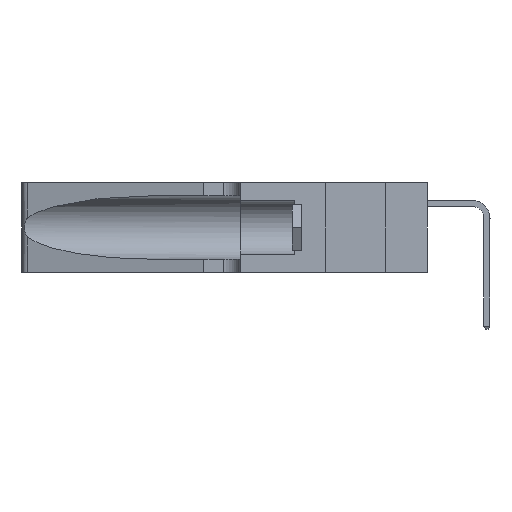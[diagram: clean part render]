
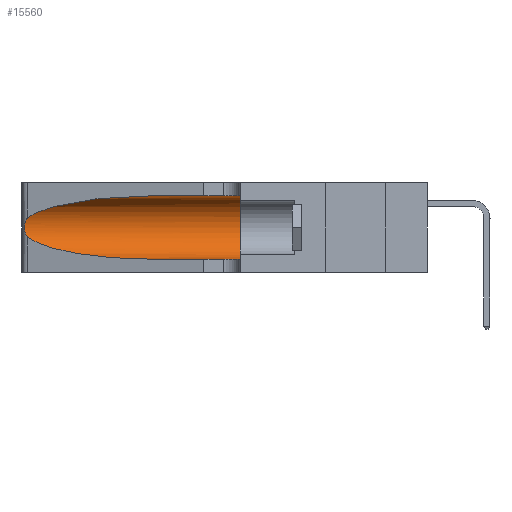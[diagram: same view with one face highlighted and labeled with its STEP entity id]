
A CAD part, left-side view. The second image highlights one B-rep face of the part: STEP entity #15560.
In plain terms, the highlighted cylindrical face has radius 3.308 mm (diameter 6.617 mm), a partial arc.
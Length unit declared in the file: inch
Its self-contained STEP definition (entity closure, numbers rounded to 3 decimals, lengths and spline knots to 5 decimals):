
#307 = CARTESIAN_POINT ( 'NONE',  ( 0.25856, 1.23593, 0.16098 ) ) ;
#1010 = EDGE_CURVE ( 'NONE', #24954, #26851, #30352, .T. ) ;
#1242 = CARTESIAN_POINT ( 'NONE',  ( 0.1305, 0.35, 0.31525 ) ) ;
#2474 = VERTEX_POINT ( 'NONE', #1242 ) ;
#3265 = CARTESIAN_POINT ( 'NONE',  ( 0.25487, 1.22718, 0.22369 ) ) ;
#3398 = CARTESIAN_POINT ( 'NONE',  ( 0.25639, 1.23186, 0.15144 ) ) ;
#3695 = DIRECTION ( 'NONE',  ( 0., 0., -1. ) ) ;
#4111 = VERTEX_POINT ( 'NONE', #16130 ) ;
#4915 = CARTESIAN_POINT ( 'NONE',  ( 0.1305, 0.72297, 0.31525 ) ) ;
#5141 = ORIENTED_EDGE ( 'NONE', *, *, #1010, .T. ) ;
#5657 = CARTESIAN_POINT ( 'NONE',  ( 0.18966, 0.96281, 0.05475 ) ) ;
#6022 = CARTESIAN_POINT ( 'NONE',  ( 0.1305, 0.72297, 0.31525 ) ) ;
#6256 = VECTOR ( 'NONE', #17718, 39.37008 ) ;
#6457 = CARTESIAN_POINT ( 'NONE',  ( 0.25487, 1.22718, 0.14631 ) ) ;
#6634 = CARTESIAN_POINT ( 'NONE',  ( 0.1305, 0.35, 0.05475 ) ) ;
#6890 = AXIS2_PLACEMENT_3D ( 'NONE', #16538, #37881, #19611 ) ;
#8808 = CIRCLE ( 'NONE', #6890, 0.13025 ) ;
#9155 = EDGE_CURVE ( 'NONE', #38205, #15535, #33438, .T. ) ;
#9383 = CARTESIAN_POINT ( 'NONE',  ( 0.25639, 1.23184, 0.21858 ) ) ;
#9835 = FACE_OUTER_BOUND ( 'NONE', #18529, .T. ) ;
#12462 = CARTESIAN_POINT ( 'NONE',  ( 0.25854, 1.2359, 0.20912 ) ) ;
#15535 = VERTEX_POINT ( 'NONE', #6634 ) ;
#15548 = CARTESIAN_POINT ( 'NONE',  ( 0.26075, 1.23896, 0.19203 ) ) ;
#15560 = ADVANCED_FACE ( 'NONE', ( #9835 ), #24211, .F. ) ;
#16130 = CARTESIAN_POINT ( 'NONE',  ( 0.25487, 1.22718, 0.14631 ) ) ;
#16538 = CARTESIAN_POINT ( 'NONE',  ( 0.1305, 0.35, 0.185 ) ) ;
#17172 = VECTOR ( 'NONE', #23485, 39.37008 ) ;
#17314 = B_SPLINE_CURVE_WITH_KNOTS ( 'NONE', 3,
 ( #3265, #21574, #9383, #30786, #12462, #33816, #15548, #36885, #18593, #307, #21700, #3398, #24771, #6457 ),
 .UNSPECIFIED., .F., .F.,
 ( 4, 2, 2, 2, 2, 2, 4 ),
 ( 0., 0.00027, 0.00053, 0.00107, 0.0016, 0.00187, 0.00214 ),
 .UNSPECIFIED. ) ;
#17718 = DIRECTION ( 'NONE',  ( 0., -1., 0. ) ) ;
#18132 = ORIENTED_EDGE ( 'NONE', *, *, #24837, .F. ) ;
#18170 = CARTESIAN_POINT ( 'NONE',  ( 0.2373, 1.15595, 0.28018 ) ) ;
#18529 = EDGE_LOOP ( 'NONE', ( #5141, #31185, #35513, #30365, #18132, #34226 ) ) ;
#18593 = CARTESIAN_POINT ( 'NONE',  ( 0.26017, 1.23833, 0.17102 ) ) ;
#19611 = DIRECTION ( 'NONE',  ( 0., 0., 1. ) ) ;
#20794 = CARTESIAN_POINT ( 'NONE',  ( 0.25487, 1.22718, 0.14631 ) ) ;
#20922 = CARTESIAN_POINT ( 'NONE',  ( 0.2373, 1.15595, 0.08982 ) ) ;
#21276 = EDGE_CURVE ( 'NONE', #4111, #38205, #25463, .T. ) ;
#21574 = CARTESIAN_POINT ( 'NONE',  ( 0.25555, 1.22994, 0.2215 ) ) ;
#21700 = CARTESIAN_POINT ( 'NONE',  ( 0.25789, 1.23486, 0.15765 ) ) ;
#22001 = DIRECTION ( 'NONE',  ( 0., -1., 0. ) ) ;
#23485 = DIRECTION ( 'NONE',  ( 0., -1., 0. ) ) ;
#23996 = EDGE_CURVE ( 'NONE', #26851, #4111, #17314, .T. ) ;
#24211 = CYLINDRICAL_SURFACE ( 'NONE', #36183, 0.13025 ) ;
#24771 = CARTESIAN_POINT ( 'NONE',  ( 0.25555, 1.22993, 0.14849 ) ) ;
#24837 = EDGE_CURVE ( 'NONE', #2474, #15535, #8808, .T. ) ;
#24954 = VERTEX_POINT ( 'NONE', #4915 ) ;
#25463 =( BOUNDED_CURVE ( )  B_SPLINE_CURVE ( 3, ( #20794, #20922, #5657, #27037 ),
 .UNSPECIFIED., .F., .F. ) 
 B_SPLINE_CURVE_WITH_KNOTS ( ( 4, 4 ),
 ( 3.44316, 4.71239 ),
 .UNSPECIFIED. ) 
 CURVE ( )  GEOMETRIC_REPRESENTATION_ITEM ( )  RATIONAL_B_SPLINE_CURVE ( ( 1., 0.87, 0.87, 1. ) ) 
 REPRESENTATION_ITEM ( '' )  );
#26851 = VERTEX_POINT ( 'NONE', #36960 ) ;
#27037 = CARTESIAN_POINT ( 'NONE',  ( 0.1305, 0.72297, 0.05475 ) ) ;
#27418 = CARTESIAN_POINT ( 'NONE',  ( 0.25487, 1.22718, 0.22369 ) ) ;
#29625 = CARTESIAN_POINT ( 'NONE',  ( 0.1305, 1.61858, 0.05475 ) ) ;
#30352 =( BOUNDED_CURVE ( )  B_SPLINE_CURVE ( 3, ( #6022, #39498, #18170, #27418 ),
 .UNSPECIFIED., .F., .T. ) 
 B_SPLINE_CURVE_WITH_KNOTS ( ( 4, 4 ),
 ( 1.5708, 2.84003 ),
 .UNSPECIFIED. ) 
 CURVE ( )  GEOMETRIC_REPRESENTATION_ITEM ( )  RATIONAL_B_SPLINE_CURVE ( ( 1., 0.87, 0.87, 1. ) ) 
 REPRESENTATION_ITEM ( '' )  );
#30365 = ORIENTED_EDGE ( 'NONE', *, *, #9155, .T. ) ;
#30659 = LINE ( 'NONE', #32963, #6256 ) ;
#30786 = CARTESIAN_POINT ( 'NONE',  ( 0.25787, 1.23484, 0.2124 ) ) ;
#31091 = CARTESIAN_POINT ( 'NONE',  ( 0.1305, 1.61858, 0.185 ) ) ;
#31185 = ORIENTED_EDGE ( 'NONE', *, *, #23996, .T. ) ;
#32006 = EDGE_CURVE ( 'NONE', #24954, #2474, #30659, .T. ) ;
#32963 = CARTESIAN_POINT ( 'NONE',  ( 0.1305, 1.61858, 0.31525 ) ) ;
#33438 = LINE ( 'NONE', #29625, #17172 ) ;
#33816 = CARTESIAN_POINT ( 'NONE',  ( 0.26018, 1.23835, 0.19895 ) ) ;
#34226 = ORIENTED_EDGE ( 'NONE', *, *, #32006, .F. ) ;
#35513 = ORIENTED_EDGE ( 'NONE', *, *, #21276, .T. ) ;
#36183 = AXIS2_PLACEMENT_3D ( 'NONE', #31091, #22001, #3695 ) ;
#36885 = CARTESIAN_POINT ( 'NONE',  ( 0.26075, 1.23896, 0.178 ) ) ;
#36960 = CARTESIAN_POINT ( 'NONE',  ( 0.25487, 1.22718, 0.22369 ) ) ;
#37881 = DIRECTION ( 'NONE',  ( 0., 1., 0. ) ) ;
#38104 = CARTESIAN_POINT ( 'NONE',  ( 0.1305, 0.72297, 0.05475 ) ) ;
#38205 = VERTEX_POINT ( 'NONE', #38104 ) ;
#39498 = CARTESIAN_POINT ( 'NONE',  ( 0.18966, 0.96281, 0.31525 ) ) ;
